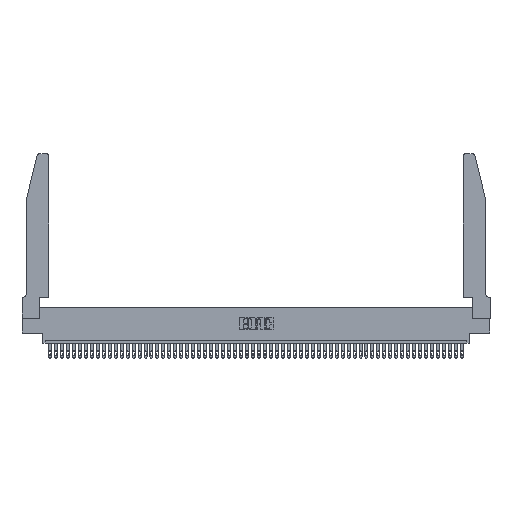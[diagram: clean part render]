
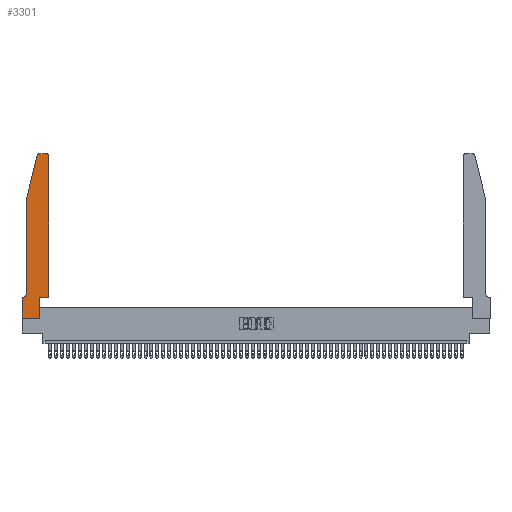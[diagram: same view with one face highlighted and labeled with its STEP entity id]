
A CAD part, top view. The second image highlights one B-rep face of the part: STEP entity #3301.
In plain terms, the highlighted planar face has unit normal (0, 0, 1).
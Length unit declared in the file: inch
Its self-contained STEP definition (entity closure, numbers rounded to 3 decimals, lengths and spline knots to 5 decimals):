
#1293 = AXIS2_PLACEMENT_3D ( 'NONE', #34961, #43462, #43284 ) ;
#1498 = CARTESIAN_POINT ( 'NONE',  ( 0.2865, 0.35, 0.37 ) ) ;
#1757 = EDGE_LOOP ( 'NONE', ( #25673, #47131, #7225, #36962, #26779, #42283, #47606, #11695, #5107, #4392, #37421, #36061 ) ) ;
#3301 = ADVANCED_FACE ( 'NONE', ( #8743 ), #35337, .T. ) ;
#3613 = VECTOR ( 'NONE', #48031, 39.37008 ) ;
#4392 = ORIENTED_EDGE ( 'NONE', *, *, #36213, .T. ) ;
#4558 = EDGE_CURVE ( 'NONE', #30882, #8860, #10856, .T. ) ;
#4810 = CIRCLE ( 'NONE', #18260, 0.03 ) ;
#5107 = ORIENTED_EDGE ( 'NONE', *, *, #4558, .T. ) ;
#5572 = DIRECTION ( 'NONE',  ( 1., 0., 0. ) ) ;
#7032 = CARTESIAN_POINT ( 'NONE',  ( 0.0755, 2., 0.37 ) ) ;
#7225 = ORIENTED_EDGE ( 'NONE', *, *, #21458, .T. ) ;
#8155 = CARTESIAN_POINT ( 'NONE',  ( 0., 0.35, 0.37 ) ) ;
#8715 = VERTEX_POINT ( 'NONE', #8155 ) ;
#8743 = FACE_OUTER_BOUND ( 'NONE', #1757, .T. ) ;
#8860 = VERTEX_POINT ( 'NONE', #1498 ) ;
#9191 = EDGE_CURVE ( 'NONE', #30792, #8715, #9648, .T. ) ;
#9648 = LINE ( 'NONE', #39603, #28677 ) ;
#9838 = CARTESIAN_POINT ( 'NONE',  ( 0.4505, 0.35, 0.37 ) ) ;
#10074 = CARTESIAN_POINT ( 'NONE',  ( 0.0055, 0.35, 0.37 ) ) ;
#10165 = CARTESIAN_POINT ( 'NONE',  ( 0.0755, 2., 0.37 ) ) ;
#10856 = LINE ( 'NONE', #11428, #12194 ) ;
#11116 = CARTESIAN_POINT ( 'NONE',  ( 0.284, 2.75, 0.37 ) ) ;
#11340 = CARTESIAN_POINT ( 'NONE',  ( 0.4205, 2.75, 0.37 ) ) ;
#11428 = CARTESIAN_POINT ( 'NONE',  ( 0.2865, 0.35, 0.37 ) ) ;
#11612 = VERTEX_POINT ( 'NONE', #11340 ) ;
#11695 = ORIENTED_EDGE ( 'NONE', *, *, #25617, .T. ) ;
#12194 = VECTOR ( 'NONE', #49104, 39.37008 ) ;
#12615 = VERTEX_POINT ( 'NONE', #33054 ) ;
#14079 = DIRECTION ( 'NONE',  ( 0., 0., 1. ) ) ;
#14929 = AXIS2_PLACEMENT_3D ( 'NONE', #32648, #28667, #20270 ) ;
#15380 = VERTEX_POINT ( 'NONE', #24169 ) ;
#16007 = LINE ( 'NONE', #49707, #30233 ) ;
#16572 = VERTEX_POINT ( 'NONE', #24010 ) ;
#17168 = LINE ( 'NONE', #44478, #27622 ) ;
#18260 = AXIS2_PLACEMENT_3D ( 'NONE', #20125, #43723, #35285 ) ;
#18277 = DIRECTION ( 'NONE',  ( 1., 0., 0. ) ) ;
#18796 = CIRCLE ( 'NONE', #26649, 0.03 ) ;
#19034 = LINE ( 'NONE', #7032, #19718 ) ;
#19718 = VECTOR ( 'NONE', #29358, 39.37008 ) ;
#20125 = CARTESIAN_POINT ( 'NONE',  ( 0.4205, 2.72, 0.37 ) ) ;
#20270 = DIRECTION ( 'NONE',  ( -1., 0., 0. ) ) ;
#21117 = EDGE_CURVE ( 'NONE', #23056, #12615, #41837, .T. ) ;
#21458 = EDGE_CURVE ( 'NONE', #37567, #16572, #26204, .T. ) ;
#23056 = VERTEX_POINT ( 'NONE', #9838 ) ;
#24010 = CARTESIAN_POINT ( 'NONE',  ( 0.0755, 2., 0.37 ) ) ;
#24169 = CARTESIAN_POINT ( 'NONE',  ( 0., 0., 0.37 ) ) ;
#24663 = CIRCLE ( 'NONE', #14929, 0.07 ) ;
#25293 = EDGE_CURVE ( 'NONE', #37290, #37567, #18796, .T. ) ;
#25393 = VECTOR ( 'NONE', #5572, 39.37008 ) ;
#25617 = EDGE_CURVE ( 'NONE', #15380, #30882, #33788, .T. ) ;
#25673 = ORIENTED_EDGE ( 'NONE', *, *, #34306, .T. ) ;
#26204 = LINE ( 'NONE', #10165, #34016 ) ;
#26649 = AXIS2_PLACEMENT_3D ( 'NONE', #43307, #14079, #18277 ) ;
#26779 = ORIENTED_EDGE ( 'NONE', *, *, #43883, .T. ) ;
#26909 = DIRECTION ( 'NONE',  ( -0.239, -0.971, 0. ) ) ;
#27622 = VECTOR ( 'NONE', #39959, 39.37008 ) ;
#28667 = DIRECTION ( 'NONE',  ( 0., 0., -1. ) ) ;
#28677 = VECTOR ( 'NONE', #43538, 39.37008 ) ;
#29358 = DIRECTION ( 'NONE',  ( 0., -1., 0. ) ) ;
#30233 = VECTOR ( 'NONE', #32767, 39.37008 ) ;
#30792 = VERTEX_POINT ( 'NONE', #10074 ) ;
#30882 = VERTEX_POINT ( 'NONE', #38782 ) ;
#32648 = CARTESIAN_POINT ( 'NONE',  ( 0.0055, 0.42, 0.37 ) ) ;
#32767 = DIRECTION ( 'NONE',  ( 0., -1., 0. ) ) ;
#33054 = CARTESIAN_POINT ( 'NONE',  ( 0.4505, 2.72, 0.37 ) ) ;
#33225 = EDGE_CURVE ( 'NONE', #16572, #36658, #19034, .T. ) ;
#33788 = LINE ( 'NONE', #38090, #25393 ) ;
#34016 = VECTOR ( 'NONE', #26909, 39.37008 ) ;
#34306 = EDGE_CURVE ( 'NONE', #11612, #37290, #43488, .T. ) ;
#34961 = CARTESIAN_POINT ( 'NONE',  ( 0., 0.35, 0.37 ) ) ;
#35285 = DIRECTION ( 'NONE',  ( 1., 0., 0. ) ) ;
#35337 = PLANE ( 'NONE',  #1293 ) ;
#35992 = CARTESIAN_POINT ( 'NONE',  ( 0.25487, 2.72718, 0.37 ) ) ;
#36061 = ORIENTED_EDGE ( 'NONE', *, *, #36092, .T. ) ;
#36092 = EDGE_CURVE ( 'NONE', #12615, #11612, #4810, .T. ) ;
#36213 = EDGE_CURVE ( 'NONE', #8860, #23056, #17168, .T. ) ;
#36658 = VERTEX_POINT ( 'NONE', #38602 ) ;
#36962 = ORIENTED_EDGE ( 'NONE', *, *, #33225, .T. ) ;
#37290 = VERTEX_POINT ( 'NONE', #11116 ) ;
#37421 = ORIENTED_EDGE ( 'NONE', *, *, #21117, .T. ) ;
#37567 = VERTEX_POINT ( 'NONE', #35992 ) ;
#37770 = DIRECTION ( 'NONE',  ( -1., 0., 0. ) ) ;
#38090 = CARTESIAN_POINT ( 'NONE',  ( 0., 0., 0.37 ) ) ;
#38602 = CARTESIAN_POINT ( 'NONE',  ( 0.0755, 0.42, 0.37 ) ) ;
#38782 = CARTESIAN_POINT ( 'NONE',  ( 0.2865, 0., 0.37 ) ) ;
#39603 = CARTESIAN_POINT ( 'NONE',  ( 0.0755, 0.35, 0.37 ) ) ;
#39959 = DIRECTION ( 'NONE',  ( 1., 0., 0. ) ) ;
#40920 = CARTESIAN_POINT ( 'NONE',  ( 0.2605, 2.75, 0.37 ) ) ;
#41715 = EDGE_CURVE ( 'NONE', #8715, #15380, #16007, .T. ) ;
#41837 = LINE ( 'NONE', #51589, #3613 ) ;
#42283 = ORIENTED_EDGE ( 'NONE', *, *, #9191, .T. ) ;
#43284 = DIRECTION ( 'NONE',  ( 1., 0., 0. ) ) ;
#43307 = CARTESIAN_POINT ( 'NONE',  ( 0.284, 2.72, 0.37 ) ) ;
#43462 = DIRECTION ( 'NONE',  ( 0., 0., 1. ) ) ;
#43488 = LINE ( 'NONE', #40920, #51894 ) ;
#43538 = DIRECTION ( 'NONE',  ( -1., 0., 0. ) ) ;
#43723 = DIRECTION ( 'NONE',  ( 0., 0., 1. ) ) ;
#43883 = EDGE_CURVE ( 'NONE', #36658, #30792, #24663, .T. ) ;
#44478 = CARTESIAN_POINT ( 'NONE',  ( 0.4505, 0.35, 0.37 ) ) ;
#47131 = ORIENTED_EDGE ( 'NONE', *, *, #25293, .T. ) ;
#47606 = ORIENTED_EDGE ( 'NONE', *, *, #41715, .T. ) ;
#48031 = DIRECTION ( 'NONE',  ( 0., 1., 0. ) ) ;
#49104 = DIRECTION ( 'NONE',  ( 0., 1., 0. ) ) ;
#49707 = CARTESIAN_POINT ( 'NONE',  ( 0., 0., 0.37 ) ) ;
#51589 = CARTESIAN_POINT ( 'NONE',  ( 0.4505, 0.35, 0.37 ) ) ;
#51894 = VECTOR ( 'NONE', #37770, 39.37008 ) ;
